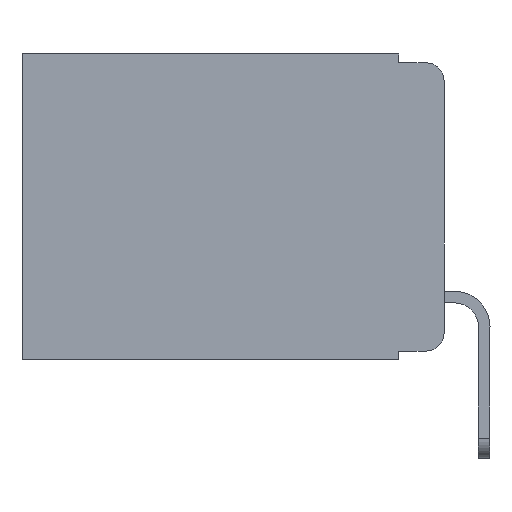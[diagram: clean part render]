
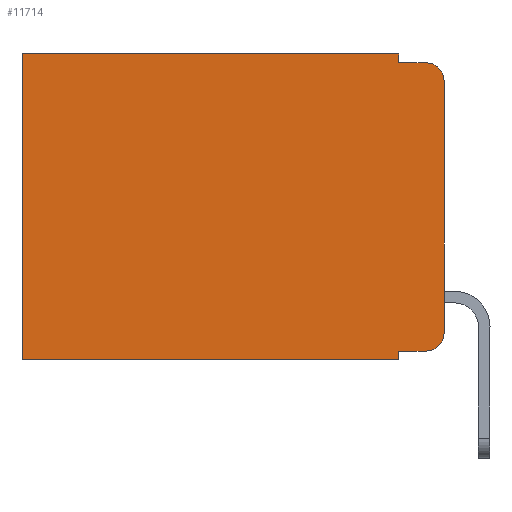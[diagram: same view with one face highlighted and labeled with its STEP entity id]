
A CAD part, left-side view. The second image highlights one B-rep face of the part: STEP entity #11714.
In plain terms, the highlighted planar face has unit normal (-1, 0, 0).
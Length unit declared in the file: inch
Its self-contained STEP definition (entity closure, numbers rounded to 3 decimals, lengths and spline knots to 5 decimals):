
#14 = DIRECTION ( 'NONE',  ( 0., 1., 0. ) ) ;
#121 = ORIENTED_EDGE ( 'NONE', *, *, #10734, .T. ) ;
#145 = EDGE_CURVE ( 'NONE', #13408, #7250, #11369, .T. ) ;
#185 = VECTOR ( 'NONE', #1044, 39.37008 ) ;
#193 = LINE ( 'NONE', #6165, #2726 ) ;
#308 = FACE_OUTER_BOUND ( 'NONE', #11404, .T. ) ;
#451 = EDGE_CURVE ( 'NONE', #5979, #7297, #10525, .T. ) ;
#782 = VERTEX_POINT ( 'NONE', #3140 ) ;
#795 = DIRECTION ( 'NONE',  ( 0., 0., -1. ) ) ;
#1044 = DIRECTION ( 'NONE',  ( 0., 0., -1. ) ) ;
#1287 = ORIENTED_EDGE ( 'NONE', *, *, #11449, .T. ) ;
#1312 = CARTESIAN_POINT ( 'NONE',  ( 0.298, 0., 0. ) ) ;
#1733 = ORIENTED_EDGE ( 'NONE', *, *, #145, .T. ) ;
#1798 = CARTESIAN_POINT ( 'NONE',  ( 0.298, 0.051, -0.01 ) ) ;
#1900 = CARTESIAN_POINT ( 'NONE',  ( 0.298, 0.051, -0.01 ) ) ;
#2033 = DIRECTION ( 'NONE',  ( -1., 0., 0. ) ) ;
#2084 = CARTESIAN_POINT ( 'NONE',  ( 0.298, 0., -0.03 ) ) ;
#2581 = AXIS2_PLACEMENT_3D ( 'NONE', #12535, #2033, #9439 ) ;
#2587 = DIRECTION ( 'NONE',  ( 0., 0., -1. ) ) ;
#2726 = VECTOR ( 'NONE', #795, 39.37008 ) ;
#2756 = EDGE_CURVE ( 'NONE', #4089, #7250, #11252, .T. ) ;
#2801 = VECTOR ( 'NONE', #14, 39.37008 ) ;
#3140 = CARTESIAN_POINT ( 'NONE',  ( 0.298, 0.051, 0. ) ) ;
#3270 = LINE ( 'NONE', #9827, #13757 ) ;
#3506 = VERTEX_POINT ( 'NONE', #8489 ) ;
#3558 = DIRECTION ( 'NONE',  ( -1., 0., 0. ) ) ;
#3779 = LINE ( 'NONE', #8326, #8598 ) ;
#3784 = CARTESIAN_POINT ( 'NONE',  ( 0.298, 0., 0. ) ) ;
#4074 = EDGE_CURVE ( 'NONE', #13408, #3506, #193, .T. ) ;
#4089 = VERTEX_POINT ( 'NONE', #1900 ) ;
#4161 = DIRECTION ( 'NONE',  ( 0., 0., -1. ) ) ;
#4489 = VERTEX_POINT ( 'NONE', #5595 ) ;
#4523 = VECTOR ( 'NONE', #8163, 39.37008 ) ;
#5246 = EDGE_CURVE ( 'NONE', #4489, #11129, #8673, .T. ) ;
#5261 = LINE ( 'NONE', #12638, #2801 ) ;
#5269 = CARTESIAN_POINT ( 'NONE',  ( 0.298, 0.051, -0.333 ) ) ;
#5595 = CARTESIAN_POINT ( 'NONE',  ( 0.298, 0.473, 0. ) ) ;
#5979 = VERTEX_POINT ( 'NONE', #5269 ) ;
#6165 = CARTESIAN_POINT ( 'NONE',  ( 0.298, 0., 0. ) ) ;
#6280 = VERTEX_POINT ( 'NONE', #9157 ) ;
#6593 = ORIENTED_EDGE ( 'NONE', *, *, #451, .T. ) ;
#6856 = EDGE_CURVE ( 'NONE', #782, #4089, #3779, .T. ) ;
#6973 = ORIENTED_EDGE ( 'NONE', *, *, #4074, .F. ) ;
#7060 = AXIS2_PLACEMENT_3D ( 'NONE', #1312, #7820, #11965 ) ;
#7250 = VERTEX_POINT ( 'NONE', #10216 ) ;
#7297 = VERTEX_POINT ( 'NONE', #8269 ) ;
#7800 = EDGE_CURVE ( 'NONE', #5979, #6280, #3270, .T. ) ;
#7820 = DIRECTION ( 'NONE',  ( 1., 0., 0. ) ) ;
#8163 = DIRECTION ( 'NONE',  ( 0., -1., 0. ) ) ;
#8203 = ORIENTED_EDGE ( 'NONE', *, *, #5246, .T. ) ;
#8269 = CARTESIAN_POINT ( 'NONE',  ( 0.298, 0.02, -0.333 ) ) ;
#8326 = CARTESIAN_POINT ( 'NONE',  ( 0.298, 0.051, 0. ) ) ;
#8489 = CARTESIAN_POINT ( 'NONE',  ( 0.298, 0., -0.313 ) ) ;
#8598 = VECTOR ( 'NONE', #4161, 39.37008 ) ;
#8673 = LINE ( 'NONE', #13736, #185 ) ;
#9157 = CARTESIAN_POINT ( 'NONE',  ( 0.298, 0.051, -0.343 ) ) ;
#9439 = DIRECTION ( 'NONE',  ( 0., 0., -1. ) ) ;
#9508 = CARTESIAN_POINT ( 'NONE',  ( 0.298, 0.473, -0.343 ) ) ;
#9633 = LINE ( 'NONE', #3784, #11150 ) ;
#9678 = DIRECTION ( 'NONE',  ( 0., 0., -1. ) ) ;
#9679 = ORIENTED_EDGE ( 'NONE', *, *, #6856, .F. ) ;
#9827 = CARTESIAN_POINT ( 'NONE',  ( 0.298, 0.051, 0. ) ) ;
#9969 = CARTESIAN_POINT ( 'NONE',  ( 0.298, 0.02, -0.313 ) ) ;
#10216 = CARTESIAN_POINT ( 'NONE',  ( 0.298, 0.02, -0.01 ) ) ;
#10293 = AXIS2_PLACEMENT_3D ( 'NONE', #9969, #3558, #2587 ) ;
#10525 = LINE ( 'NONE', #13498, #4523 ) ;
#10734 = EDGE_CURVE ( 'NONE', #7297, #3506, #12644, .T. ) ;
#11046 = PLANE ( 'NONE',  #7060 ) ;
#11129 = VERTEX_POINT ( 'NONE', #9508 ) ;
#11143 = ORIENTED_EDGE ( 'NONE', *, *, #7800, .F. ) ;
#11150 = VECTOR ( 'NONE', #11244, 39.37008 ) ;
#11244 = DIRECTION ( 'NONE',  ( 0., 1., 0. ) ) ;
#11252 = LINE ( 'NONE', #1798, #11415 ) ;
#11296 = DIRECTION ( 'NONE',  ( 0., -1., 0. ) ) ;
#11369 = CIRCLE ( 'NONE', #2581, 0.02 ) ;
#11404 = EDGE_LOOP ( 'NONE', ( #6973, #1733, #11503, #9679, #1287, #8203, #12661, #11143, #6593, #121 ) ) ;
#11415 = VECTOR ( 'NONE', #11296, 39.37008 ) ;
#11449 = EDGE_CURVE ( 'NONE', #782, #4489, #9633, .T. ) ;
#11503 = ORIENTED_EDGE ( 'NONE', *, *, #2756, .F. ) ;
#11714 = ADVANCED_FACE ( 'NONE', ( #308 ), #11046, .F. ) ;
#11965 = DIRECTION ( 'NONE',  ( 0., 0., -1. ) ) ;
#12535 = CARTESIAN_POINT ( 'NONE',  ( 0.298, 0.02, -0.03 ) ) ;
#12638 = CARTESIAN_POINT ( 'NONE',  ( 0.298, 0., -0.343 ) ) ;
#12644 = CIRCLE ( 'NONE', #10293, 0.02 ) ;
#12661 = ORIENTED_EDGE ( 'NONE', *, *, #12743, .F. ) ;
#12743 = EDGE_CURVE ( 'NONE', #6280, #11129, #5261, .T. ) ;
#13408 = VERTEX_POINT ( 'NONE', #2084 ) ;
#13498 = CARTESIAN_POINT ( 'NONE',  ( 0.298, 0.051, -0.333 ) ) ;
#13736 = CARTESIAN_POINT ( 'NONE',  ( 0.298, 0.473, 0. ) ) ;
#13757 = VECTOR ( 'NONE', #9678, 39.37008 ) ;
